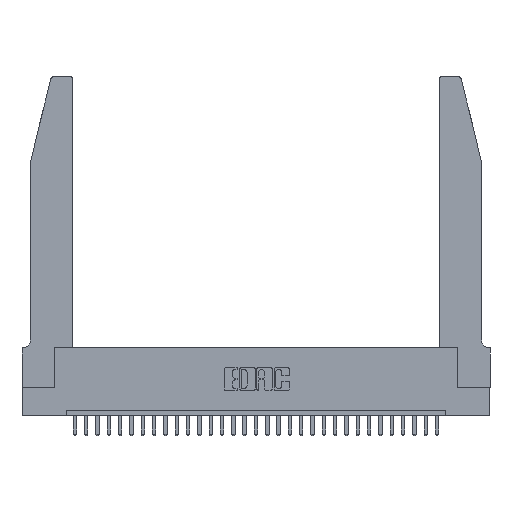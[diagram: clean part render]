
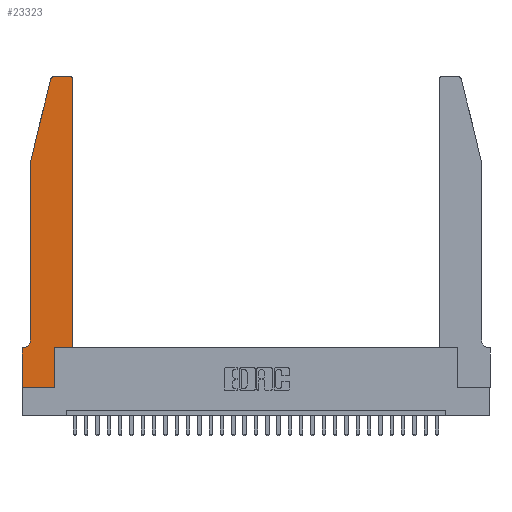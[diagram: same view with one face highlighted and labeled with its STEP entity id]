
A CAD part, top view. The second image highlights one B-rep face of the part: STEP entity #23323.
In plain terms, the highlighted planar face has unit normal (0, 0, 1).
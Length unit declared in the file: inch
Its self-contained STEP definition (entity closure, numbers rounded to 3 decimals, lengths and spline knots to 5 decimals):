
#1250 = EDGE_CURVE ( 'NONE', #16241, #25925, #30830, .T. ) ;
#1797 = ORIENTED_EDGE ( 'NONE', *, *, #7619, .T. ) ;
#1915 = CARTESIAN_POINT ( 'NONE',  ( 0.284, 2.72, 0.37 ) ) ;
#2008 = VECTOR ( 'NONE', #25360, 39.37008 ) ;
#2277 = VECTOR ( 'NONE', #17378, 39.37008 ) ;
#2508 = EDGE_CURVE ( 'NONE', #7012, #21686, #24771, .T. ) ;
#3021 = LINE ( 'NONE', #21829, #3743 ) ;
#3037 = ORIENTED_EDGE ( 'NONE', *, *, #23630, .T. ) ;
#3089 = CARTESIAN_POINT ( 'NONE',  ( 0.0755, 2., 0.37 ) ) ;
#3395 = FACE_OUTER_BOUND ( 'NONE', #15381, .T. ) ;
#3531 = VERTEX_POINT ( 'NONE', #13980 ) ;
#3743 = VECTOR ( 'NONE', #19323, 39.37008 ) ;
#3906 = VERTEX_POINT ( 'NONE', #24695 ) ;
#4520 = LINE ( 'NONE', #7715, #2277 ) ;
#4529 = DIRECTION ( 'NONE',  ( 0., 0., 1. ) ) ;
#5375 = CARTESIAN_POINT ( 'NONE',  ( 0.0755, 0.35, 0.37 ) ) ;
#5491 = CIRCLE ( 'NONE', #8084, 0.03 ) ;
#6461 = CARTESIAN_POINT ( 'NONE',  ( 0.2865, 0.35, 0.37 ) ) ;
#6635 = CIRCLE ( 'NONE', #26729, 0.03 ) ;
#6961 = ORIENTED_EDGE ( 'NONE', *, *, #21394, .T. ) ;
#7012 = VERTEX_POINT ( 'NONE', #24394 ) ;
#7596 = DIRECTION ( 'NONE',  ( -1., 0., 0. ) ) ;
#7619 = EDGE_CURVE ( 'NONE', #21686, #30939, #8400, .T. ) ;
#7715 = CARTESIAN_POINT ( 'NONE',  ( 0., 0., 0.37 ) ) ;
#7721 = DIRECTION ( 'NONE',  ( -0.239, -0.971, 0. ) ) ;
#7796 = VERTEX_POINT ( 'NONE', #19412 ) ;
#7797 = ORIENTED_EDGE ( 'NONE', *, *, #26029, .T. ) ;
#7975 = ORIENTED_EDGE ( 'NONE', *, *, #18369, .T. ) ;
#8084 = AXIS2_PLACEMENT_3D ( 'NONE', #9428, #21148, #16807 ) ;
#8143 = VERTEX_POINT ( 'NONE', #22131 ) ;
#8400 = LINE ( 'NONE', #30064, #2008 ) ;
#8831 = PLANE ( 'NONE',  #19961 ) ;
#9096 = VECTOR ( 'NONE', #21032, 39.37008 ) ;
#9174 = CARTESIAN_POINT ( 'NONE',  ( 0.0755, 0.42, 0.37 ) ) ;
#9258 = ORIENTED_EDGE ( 'NONE', *, *, #24139, .T. ) ;
#9342 = LINE ( 'NONE', #3089, #14929 ) ;
#9372 = LINE ( 'NONE', #21155, #13846 ) ;
#9428 = CARTESIAN_POINT ( 'NONE',  ( 0.4205, 2.72, 0.37 ) ) ;
#9685 = CARTESIAN_POINT ( 'NONE',  ( 0.0055, 0.42, 0.37 ) ) ;
#10497 = CARTESIAN_POINT ( 'NONE',  ( 0.4505, 0.35, 0.37 ) ) ;
#10540 = VERTEX_POINT ( 'NONE', #22047 ) ;
#10988 = ORIENTED_EDGE ( 'NONE', *, *, #12843, .T. ) ;
#11583 = EDGE_CURVE ( 'NONE', #8143, #22982, #12376, .T. ) ;
#12073 = DIRECTION ( 'NONE',  ( -1., 0., 0. ) ) ;
#12376 = LINE ( 'NONE', #24422, #29202 ) ;
#12843 = EDGE_CURVE ( 'NONE', #26318, #8143, #9342, .T. ) ;
#13143 = AXIS2_PLACEMENT_3D ( 'NONE', #9685, #21517, #12073 ) ;
#13519 = DIRECTION ( 'NONE',  ( 1., 0., 0. ) ) ;
#13771 = CARTESIAN_POINT ( 'NONE',  ( 0.4205, 2.75, 0.37 ) ) ;
#13846 = VECTOR ( 'NONE', #23602, 39.37008 ) ;
#13874 = CARTESIAN_POINT ( 'NONE',  ( 0.25487, 2.72718, 0.37 ) ) ;
#13980 = CARTESIAN_POINT ( 'NONE',  ( 0., 0.35, 0.37 ) ) ;
#14929 = VECTOR ( 'NONE', #7721, 39.37008 ) ;
#15381 = EDGE_LOOP ( 'NONE', ( #25060, #19475, #10988, #21337, #17483, #7975, #9258, #6961, #23436, #1797, #3037, #7797 ) ) ;
#16241 = VERTEX_POINT ( 'NONE', #13771 ) ;
#16807 = DIRECTION ( 'NONE',  ( 1., 0., 0. ) ) ;
#17378 = DIRECTION ( 'NONE',  ( 1., 0., 0. ) ) ;
#17422 = VECTOR ( 'NONE', #7596, 39.37008 ) ;
#17483 = ORIENTED_EDGE ( 'NONE', *, *, #30544, .T. ) ;
#18109 = VECTOR ( 'NONE', #30608, 39.37008 ) ;
#18124 = EDGE_CURVE ( 'NONE', #25925, #26318, #6635, .T. ) ;
#18369 = EDGE_CURVE ( 'NONE', #10540, #3531, #23783, .T. ) ;
#18504 = CARTESIAN_POINT ( 'NONE',  ( 0., 0.35, 0.37 ) ) ;
#18508 = DIRECTION ( 'NONE',  ( 1., 0., 0. ) ) ;
#18809 = CARTESIAN_POINT ( 'NONE',  ( 0.2865, 0.35, 0.37 ) ) ;
#19323 = DIRECTION ( 'NONE',  ( 0., 1., 0. ) ) ;
#19412 = CARTESIAN_POINT ( 'NONE',  ( 0.4505, 2.72, 0.37 ) ) ;
#19475 = ORIENTED_EDGE ( 'NONE', *, *, #18124, .T. ) ;
#19496 = DIRECTION ( 'NONE',  ( 0., -1., 0. ) ) ;
#19961 = AXIS2_PLACEMENT_3D ( 'NONE', #18504, #23201, #13519 ) ;
#21032 = DIRECTION ( 'NONE',  ( 0., 1., 0. ) ) ;
#21148 = DIRECTION ( 'NONE',  ( 0., 0., 1. ) ) ;
#21155 = CARTESIAN_POINT ( 'NONE',  ( 0., 0., 0.37 ) ) ;
#21337 = ORIENTED_EDGE ( 'NONE', *, *, #11583, .T. ) ;
#21394 = EDGE_CURVE ( 'NONE', #3906, #7012, #4520, .T. ) ;
#21517 = DIRECTION ( 'NONE',  ( 0., 0., -1. ) ) ;
#21686 = VERTEX_POINT ( 'NONE', #18809 ) ;
#21829 = CARTESIAN_POINT ( 'NONE',  ( 0.4505, 0.35, 0.37 ) ) ;
#22047 = CARTESIAN_POINT ( 'NONE',  ( 0.0055, 0.35, 0.37 ) ) ;
#22131 = CARTESIAN_POINT ( 'NONE',  ( 0.0755, 2., 0.37 ) ) ;
#22982 = VERTEX_POINT ( 'NONE', #9174 ) ;
#23096 = CIRCLE ( 'NONE', #13143, 0.07 ) ;
#23201 = DIRECTION ( 'NONE',  ( 0., 0., 1. ) ) ;
#23323 = ADVANCED_FACE ( 'NONE', ( #3395 ), #8831, .T. ) ;
#23436 = ORIENTED_EDGE ( 'NONE', *, *, #2508, .T. ) ;
#23602 = DIRECTION ( 'NONE',  ( 0., -1., 0. ) ) ;
#23630 = EDGE_CURVE ( 'NONE', #30939, #7796, #3021, .T. ) ;
#23783 = LINE ( 'NONE', #5375, #17422 ) ;
#24139 = EDGE_CURVE ( 'NONE', #3531, #3906, #9372, .T. ) ;
#24394 = CARTESIAN_POINT ( 'NONE',  ( 0.2865, 0., 0.37 ) ) ;
#24422 = CARTESIAN_POINT ( 'NONE',  ( 0.0755, 2., 0.37 ) ) ;
#24695 = CARTESIAN_POINT ( 'NONE',  ( 0., 0., 0.37 ) ) ;
#24771 = LINE ( 'NONE', #6461, #9096 ) ;
#25060 = ORIENTED_EDGE ( 'NONE', *, *, #1250, .T. ) ;
#25360 = DIRECTION ( 'NONE',  ( 1., 0., 0. ) ) ;
#25908 = CARTESIAN_POINT ( 'NONE',  ( 0.284, 2.75, 0.37 ) ) ;
#25925 = VERTEX_POINT ( 'NONE', #25908 ) ;
#26029 = EDGE_CURVE ( 'NONE', #7796, #16241, #5491, .T. ) ;
#26318 = VERTEX_POINT ( 'NONE', #13874 ) ;
#26729 = AXIS2_PLACEMENT_3D ( 'NONE', #1915, #4529, #18508 ) ;
#28314 = CARTESIAN_POINT ( 'NONE',  ( 0.2605, 2.75, 0.37 ) ) ;
#29202 = VECTOR ( 'NONE', #19496, 39.37008 ) ;
#30064 = CARTESIAN_POINT ( 'NONE',  ( 0.4505, 0.35, 0.37 ) ) ;
#30544 = EDGE_CURVE ( 'NONE', #22982, #10540, #23096, .T. ) ;
#30608 = DIRECTION ( 'NONE',  ( -1., 0., 0. ) ) ;
#30830 = LINE ( 'NONE', #28314, #18109 ) ;
#30939 = VERTEX_POINT ( 'NONE', #10497 ) ;
